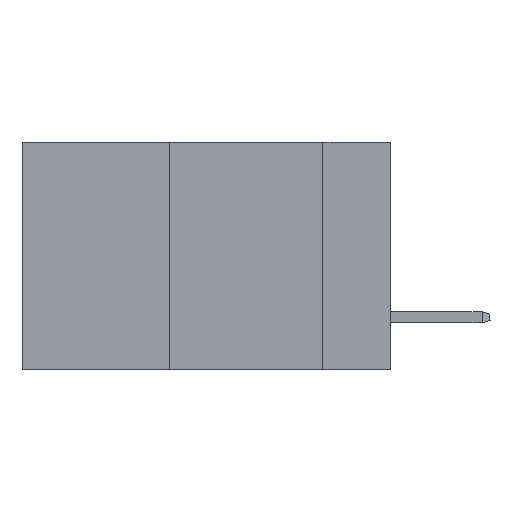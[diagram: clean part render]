
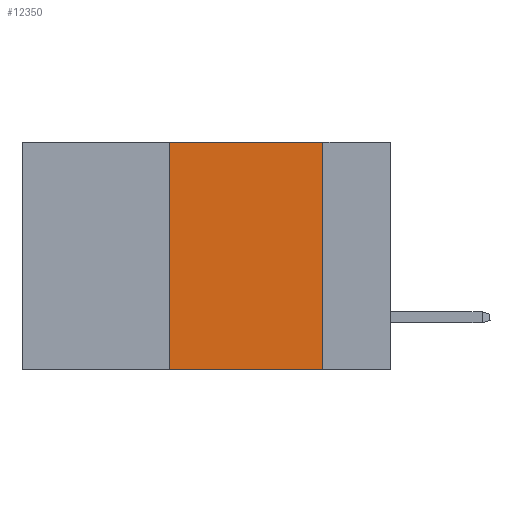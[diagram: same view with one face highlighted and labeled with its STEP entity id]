
A CAD part, left-side view. The second image highlights one B-rep face of the part: STEP entity #12350.
In plain terms, the highlighted planar face has unit normal (-1, 0, 0).
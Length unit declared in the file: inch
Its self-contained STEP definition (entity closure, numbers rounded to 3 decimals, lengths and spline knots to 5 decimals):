
#442 = CARTESIAN_POINT ( 'NONE',  ( 0., 0.6, -0.37 ) ) ;
#926 = ORIENTED_EDGE ( 'NONE', *, *, #2334, .T. ) ;
#1618 = CARTESIAN_POINT ( 'NONE',  ( 0., 0.11, 0. ) ) ;
#2334 = EDGE_CURVE ( 'NONE', #3675, #8526, #17918, .T. ) ;
#2843 = VECTOR ( 'NONE', #14165, 39.37008 ) ;
#2868 = DIRECTION ( 'NONE',  ( 0., -1., 0. ) ) ;
#3031 = CARTESIAN_POINT ( 'NONE',  ( 0., 0.11, 0. ) ) ;
#3290 = VERTEX_POINT ( 'NONE', #1618 ) ;
#3675 = VERTEX_POINT ( 'NONE', #19477 ) ;
#5948 = VECTOR ( 'NONE', #2868, 39.37008 ) ;
#6929 = DIRECTION ( 'NONE',  ( 0., -1., 0. ) ) ;
#7879 = LINE ( 'NONE', #25807, #21780 ) ;
#7893 = LINE ( 'NONE', #22955, #5948 ) ;
#8526 = VERTEX_POINT ( 'NONE', #24659 ) ;
#10527 = EDGE_LOOP ( 'NONE', ( #13794, #15947, #21277, #926 ) ) ;
#11299 = EDGE_CURVE ( 'NONE', #3290, #8526, #22822, .T. ) ;
#11895 = EDGE_CURVE ( 'NONE', #3675, #15562, #7879, .T. ) ;
#12350 = ADVANCED_FACE ( 'NONE', ( #27913 ), #28061, .F. ) ;
#13794 = ORIENTED_EDGE ( 'NONE', *, *, #11299, .F. ) ;
#14165 = DIRECTION ( 'NONE',  ( 0., 0., -1. ) ) ;
#15397 = VECTOR ( 'NONE', #6929, 39.37008 ) ;
#15562 = VERTEX_POINT ( 'NONE', #25838 ) ;
#15947 = ORIENTED_EDGE ( 'NONE', *, *, #28406, .F. ) ;
#16563 = DIRECTION ( 'NONE',  ( 0., 0., 1. ) ) ;
#16805 = CARTESIAN_POINT ( 'NONE',  ( 0., 0.6, 0. ) ) ;
#17097 = DIRECTION ( 'NONE',  ( 1., 0., 0. ) ) ;
#17918 = LINE ( 'NONE', #442, #15397 ) ;
#19477 = CARTESIAN_POINT ( 'NONE',  ( 0., 0.36, -0.37 ) ) ;
#20412 = AXIS2_PLACEMENT_3D ( 'NONE', #16805, #17097, #25772 ) ;
#21277 = ORIENTED_EDGE ( 'NONE', *, *, #11895, .F. ) ;
#21780 = VECTOR ( 'NONE', #16563, 39.37008 ) ;
#22822 = LINE ( 'NONE', #3031, #2843 ) ;
#22955 = CARTESIAN_POINT ( 'NONE',  ( 0., 0.6, 0. ) ) ;
#24659 = CARTESIAN_POINT ( 'NONE',  ( 0., 0.11, -0.37 ) ) ;
#25772 = DIRECTION ( 'NONE',  ( 0., 0., -1. ) ) ;
#25807 = CARTESIAN_POINT ( 'NONE',  ( 0., 0.36, 0. ) ) ;
#25838 = CARTESIAN_POINT ( 'NONE',  ( 0., 0.36, 0. ) ) ;
#27913 = FACE_OUTER_BOUND ( 'NONE', #10527, .T. ) ;
#28061 = PLANE ( 'NONE',  #20412 ) ;
#28406 = EDGE_CURVE ( 'NONE', #15562, #3290, #7893, .T. ) ;
